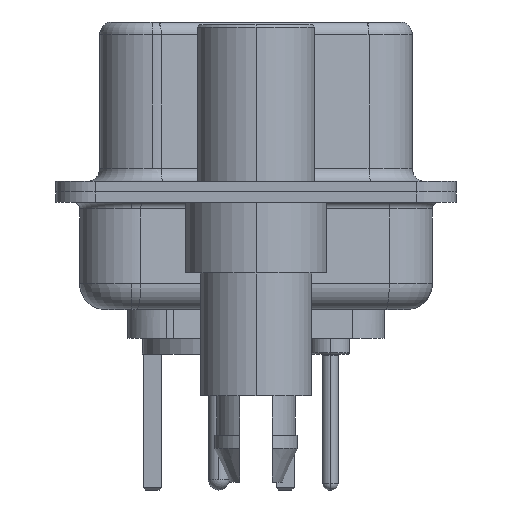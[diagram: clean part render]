
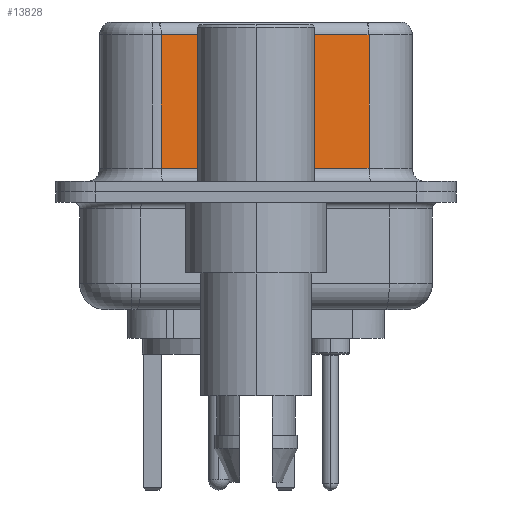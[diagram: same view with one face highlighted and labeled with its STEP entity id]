
A CAD part, left-side view. The second image highlights one B-rep face of the part: STEP entity #13828.
In plain terms, the highlighted planar face has unit normal (-0.985, -0.174, 0).
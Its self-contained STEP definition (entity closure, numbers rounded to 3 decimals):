
#1219 = CARTESIAN_POINT ( 'NONE',  ( 5.132, -4.322, 6.02 ) ) ;
#2400 = PLANE ( 'NONE',  #22987 ) ;
#3275 = CARTESIAN_POINT ( 'NONE',  ( 5.132, -4.322, 6.02 ) ) ;
#3388 = VERTEX_POINT ( 'NONE', #16103 ) ;
#4399 = ORIENTED_EDGE ( 'NONE', *, *, #26648, .T. ) ;
#4502 = VECTOR ( 'NONE', #22670, 1000. ) ;
#4522 = CARTESIAN_POINT ( 'NONE',  ( 5.132, -4.322, 6.52 ) ) ;
#4583 = DIRECTION ( 'NONE',  ( -0.174, 0.985, 0. ) ) ;
#4634 = FACE_OUTER_BOUND ( 'NONE', #13491, .T. ) ;
#4742 = DIRECTION ( 'NONE',  ( 0., 0., -1. ) ) ;
#5773 = DIRECTION ( 'NONE',  ( 0., 0., -1. ) ) ;
#6387 = VECTOR ( 'NONE', #5773, 1000. ) ;
#6724 = VERTEX_POINT ( 'NONE', #21168 ) ;
#7631 = LINE ( 'NONE', #1219, #23734 ) ;
#7994 = VECTOR ( 'NONE', #4742, 1000. ) ;
#11155 = ORIENTED_EDGE ( 'NONE', *, *, #12931, .T. ) ;
#11941 = LINE ( 'NONE', #22514, #6387 ) ;
#12161 = CARTESIAN_POINT ( 'NONE',  ( 5.132, -4.322, 0.9 ) ) ;
#12569 = ORIENTED_EDGE ( 'NONE', *, *, #17393, .T. ) ;
#12931 = EDGE_CURVE ( 'NONE', #14589, #6724, #7631, .T. ) ;
#13491 = EDGE_LOOP ( 'NONE', ( #22121, #11155, #12569, #4399 ) ) ;
#13828 = ADVANCED_FACE ( 'NONE', ( #4634 ), #2400, .F. ) ;
#14589 = VERTEX_POINT ( 'NONE', #3275 ) ;
#15999 = DIRECTION ( 'NONE',  ( -0.174, 0.985, 0. ) ) ;
#16103 = CARTESIAN_POINT ( 'NONE',  ( 3.73, 3.628, 0.9 ) ) ;
#17159 = DIRECTION ( 'NONE',  ( 0.985, 0.174, 0. ) ) ;
#17326 = CARTESIAN_POINT ( 'NONE',  ( 5.132, -4.322, 6.52 ) ) ;
#17393 = EDGE_CURVE ( 'NONE', #6724, #3388, #11941, .T. ) ;
#18795 = EDGE_CURVE ( 'NONE', #14589, #26156, #19212, .T. ) ;
#19212 = LINE ( 'NONE', #17326, #7994 ) ;
#20580 = LINE ( 'NONE', #12161, #4502 ) ;
#21168 = CARTESIAN_POINT ( 'NONE',  ( 3.73, 3.628, 6.02 ) ) ;
#21170 = CARTESIAN_POINT ( 'NONE',  ( 5.132, -4.322, 0.9 ) ) ;
#22121 = ORIENTED_EDGE ( 'NONE', *, *, #18795, .F. ) ;
#22514 = CARTESIAN_POINT ( 'NONE',  ( 3.73, 3.628, 6.52 ) ) ;
#22670 = DIRECTION ( 'NONE',  ( 0.174, -0.985, 0. ) ) ;
#22987 = AXIS2_PLACEMENT_3D ( 'NONE', #4522, #17159, #4583 ) ;
#23734 = VECTOR ( 'NONE', #15999, 1000. ) ;
#26156 = VERTEX_POINT ( 'NONE', #21170 ) ;
#26648 = EDGE_CURVE ( 'NONE', #3388, #26156, #20580, .T. ) ;
